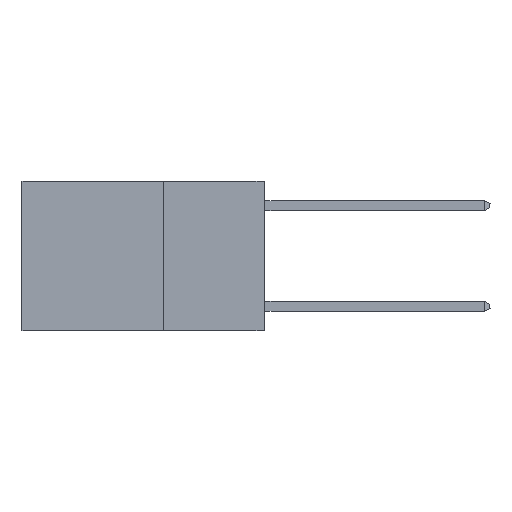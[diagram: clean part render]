
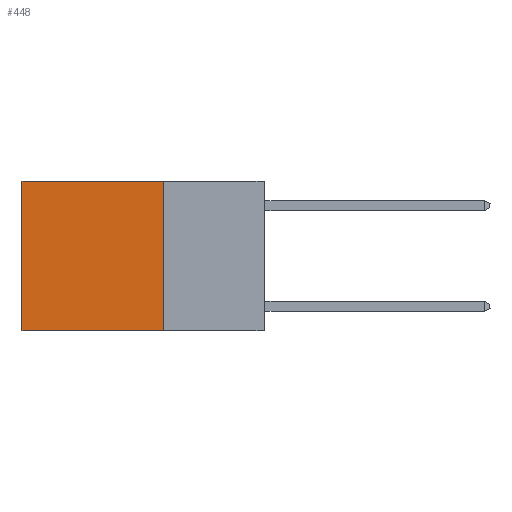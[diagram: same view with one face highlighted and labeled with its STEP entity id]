
A CAD part, left-side view. The second image highlights one B-rep face of the part: STEP entity #448.
In plain terms, the highlighted planar face has unit normal (-1, 0, 0).
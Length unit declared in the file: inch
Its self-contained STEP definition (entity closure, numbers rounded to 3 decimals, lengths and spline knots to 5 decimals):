
#448 = ADVANCED_FACE ( 'NONE', ( #19684 ), #8515, .F. ) ;
#1146 = VERTEX_POINT ( 'NONE', #10391 ) ;
#1255 = ORIENTED_EDGE ( 'NONE', *, *, #19841, .T. ) ;
#1833 = LINE ( 'NONE', #5745, #13812 ) ;
#1836 = LINE ( 'NONE', #22463, #5874 ) ;
#3441 = ORIENTED_EDGE ( 'NONE', *, *, #11980, .F. ) ;
#3579 = DIRECTION ( 'NONE',  ( 0., 0., -1. ) ) ;
#4727 = DIRECTION ( 'NONE',  ( 1., 0., 0. ) ) ;
#4851 = CARTESIAN_POINT ( 'NONE',  ( 0.2625, 0.25, -0.37 ) ) ;
#4971 = ORIENTED_EDGE ( 'NONE', *, *, #9744, .T. ) ;
#5058 = DIRECTION ( 'NONE',  ( 0., 1., 0. ) ) ;
#5745 = CARTESIAN_POINT ( 'NONE',  ( 0.2625, 0.25, 0. ) ) ;
#5874 = VECTOR ( 'NONE', #3579, 39.37008 ) ;
#6889 = VECTOR ( 'NONE', #10580, 39.37008 ) ;
#8076 = VERTEX_POINT ( 'NONE', #4851 ) ;
#8293 = VERTEX_POINT ( 'NONE', #12886 ) ;
#8515 = PLANE ( 'NONE',  #20967 ) ;
#9744 = EDGE_CURVE ( 'NONE', #23699, #8293, #1833, .T. ) ;
#9881 = CARTESIAN_POINT ( 'NONE',  ( 0.2625, 0.25, 0. ) ) ;
#10391 = CARTESIAN_POINT ( 'NONE',  ( 0.2625, 0.6, -0.37 ) ) ;
#10580 = DIRECTION ( 'NONE',  ( 0., 0., -1. ) ) ;
#10844 = CARTESIAN_POINT ( 'NONE',  ( 0.2625, 0.25, -0.37 ) ) ;
#11980 = EDGE_CURVE ( 'NONE', #8076, #1146, #16597, .T. ) ;
#12475 = CARTESIAN_POINT ( 'NONE',  ( 0.2625, 0.25, 0. ) ) ;
#12886 = CARTESIAN_POINT ( 'NONE',  ( 0.2625, 0.6, 0. ) ) ;
#13414 = DIRECTION ( 'NONE',  ( 0., 1., 0. ) ) ;
#13812 = VECTOR ( 'NONE', #13414, 39.37008 ) ;
#14463 = LINE ( 'NONE', #12475, #6889 ) ;
#16153 = CARTESIAN_POINT ( 'NONE',  ( 0.2625, 0.25, 0. ) ) ;
#16597 = LINE ( 'NONE', #10844, #17990 ) ;
#16638 = EDGE_CURVE ( 'NONE', #23699, #8076, #14463, .T. ) ;
#17220 = ORIENTED_EDGE ( 'NONE', *, *, #16638, .F. ) ;
#17990 = VECTOR ( 'NONE', #5058, 39.37008 ) ;
#18583 = EDGE_LOOP ( 'NONE', ( #1255, #3441, #17220, #4971 ) ) ;
#19684 = FACE_OUTER_BOUND ( 'NONE', #18583, .T. ) ;
#19841 = EDGE_CURVE ( 'NONE', #8293, #1146, #1836, .T. ) ;
#20064 = DIRECTION ( 'NONE',  ( 0., 0., -1. ) ) ;
#20967 = AXIS2_PLACEMENT_3D ( 'NONE', #16153, #4727, #20064 ) ;
#22463 = CARTESIAN_POINT ( 'NONE',  ( 0.2625, 0.6, 0. ) ) ;
#23699 = VERTEX_POINT ( 'NONE', #9881 ) ;
